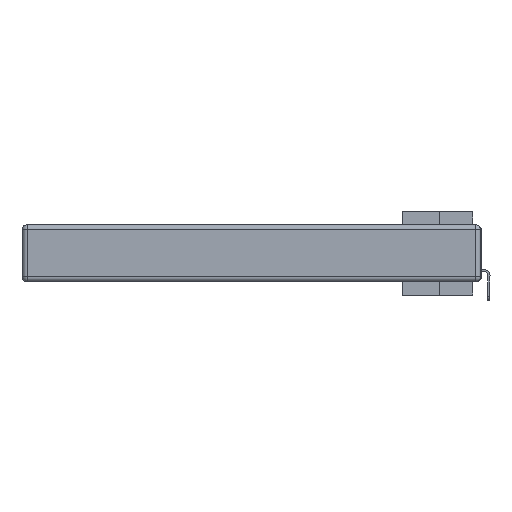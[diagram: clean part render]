
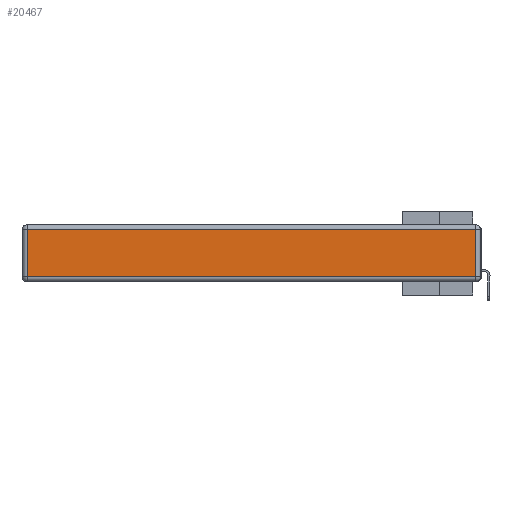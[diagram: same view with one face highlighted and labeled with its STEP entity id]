
A CAD part, left-side view. The second image highlights one B-rep face of the part: STEP entity #20467.
In plain terms, the highlighted planar face has unit normal (-1, 0, 0).
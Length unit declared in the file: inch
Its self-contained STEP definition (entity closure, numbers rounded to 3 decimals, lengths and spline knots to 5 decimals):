
#4292 = CARTESIAN_POINT ( 'NONE',  ( 0., 2.72, -0.343 ) ) ;
#4561 = VECTOR ( 'NONE', #32628, 39.37008 ) ;
#5883 = CARTESIAN_POINT ( 'NONE',  ( 0., 2.75, -0.03 ) ) ;
#6151 = ORIENTED_EDGE ( 'NONE', *, *, #14536, .T. ) ;
#6411 = LINE ( 'NONE', #9761, #10483 ) ;
#7927 = CARTESIAN_POINT ( 'NONE',  ( 0., 0.03, -0.03 ) ) ;
#8567 = EDGE_CURVE ( 'NONE', #18727, #32878, #31613, .T. ) ;
#8849 = VECTOR ( 'NONE', #25485, 39.37008 ) ;
#9729 = VECTOR ( 'NONE', #19181, 39.37008 ) ;
#9761 = CARTESIAN_POINT ( 'NONE',  ( 0., 0.03, -0.343 ) ) ;
#9970 = CARTESIAN_POINT ( 'NONE',  ( 0., 0., -0.343 ) ) ;
#10483 = VECTOR ( 'NONE', #22681, 39.37008 ) ;
#10564 = AXIS2_PLACEMENT_3D ( 'NONE', #9970, #30899, #23129 ) ;
#13911 = ORIENTED_EDGE ( 'NONE', *, *, #8567, .T. ) ;
#14536 = EDGE_CURVE ( 'NONE', #31932, #18727, #15919, .T. ) ;
#15038 = CARTESIAN_POINT ( 'NONE',  ( 0., 0., -0.313 ) ) ;
#15919 = LINE ( 'NONE', #4292, #4561 ) ;
#18727 = VERTEX_POINT ( 'NONE', #24320 ) ;
#19181 = DIRECTION ( 'NONE',  ( 0., 1., 0. ) ) ;
#19502 = LINE ( 'NONE', #5883, #9729 ) ;
#20205 = PLANE ( 'NONE',  #10564 ) ;
#20467 = ADVANCED_FACE ( 'NONE', ( #27227 ), #20205, .T. ) ;
#21267 = EDGE_CURVE ( 'NONE', #32878, #29542, #6411, .T. ) ;
#22632 = ORIENTED_EDGE ( 'NONE', *, *, #21267, .T. ) ;
#22681 = DIRECTION ( 'NONE',  ( 0., 0., 1. ) ) ;
#23129 = DIRECTION ( 'NONE',  ( 0., 0., 1. ) ) ;
#23406 = EDGE_CURVE ( 'NONE', #29542, #31932, #19502, .T. ) ;
#24320 = CARTESIAN_POINT ( 'NONE',  ( 0., 2.72, -0.313 ) ) ;
#25485 = DIRECTION ( 'NONE',  ( 0., -1., 0. ) ) ;
#26338 = CARTESIAN_POINT ( 'NONE',  ( 0., 0.03, -0.313 ) ) ;
#27227 = FACE_OUTER_BOUND ( 'NONE', #32621, .T. ) ;
#27262 = ORIENTED_EDGE ( 'NONE', *, *, #23406, .T. ) ;
#28494 = CARTESIAN_POINT ( 'NONE',  ( 0., 2.72, -0.03 ) ) ;
#29542 = VERTEX_POINT ( 'NONE', #7927 ) ;
#30899 = DIRECTION ( 'NONE',  ( -1., 0., 0. ) ) ;
#31613 = LINE ( 'NONE', #15038, #8849 ) ;
#31932 = VERTEX_POINT ( 'NONE', #28494 ) ;
#32621 = EDGE_LOOP ( 'NONE', ( #13911, #22632, #27262, #6151 ) ) ;
#32628 = DIRECTION ( 'NONE',  ( 0., 0., -1. ) ) ;
#32878 = VERTEX_POINT ( 'NONE', #26338 ) ;
